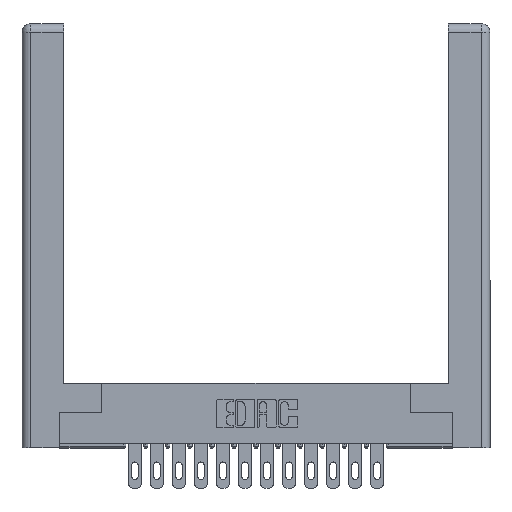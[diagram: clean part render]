
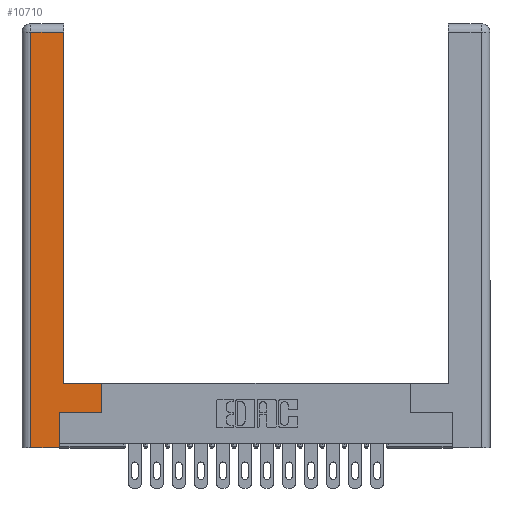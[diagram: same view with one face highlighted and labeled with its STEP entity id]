
A CAD part, top view. The second image highlights one B-rep face of the part: STEP entity #10710.
In plain terms, the highlighted planar face has unit normal (0, 0, 1).
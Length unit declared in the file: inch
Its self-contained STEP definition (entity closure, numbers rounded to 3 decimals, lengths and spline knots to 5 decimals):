
#249 = LINE ( 'NONE', #18550, #14050 ) ;
#365 = LINE ( 'NONE', #11459, #13001 ) ;
#536 = ORIENTED_EDGE ( 'NONE', *, *, #5729, .T. ) ;
#1111 = LINE ( 'NONE', #8922, #12558 ) ;
#1898 = VECTOR ( 'NONE', #13755, 39.37008 ) ;
#2188 = VERTEX_POINT ( 'NONE', #16757 ) ;
#2246 = DIRECTION ( 'NONE',  ( 0., -1., 0. ) ) ;
#2327 = CARTESIAN_POINT ( 'NONE',  ( 0.265, 0.245, 0. ) ) ;
#2480 = EDGE_CURVE ( 'NONE', #4281, #11758, #11964, .T. ) ;
#2519 = CARTESIAN_POINT ( 'NONE',  ( 0.565, 0.45, 0. ) ) ;
#2804 = EDGE_CURVE ( 'NONE', #11758, #7143, #9350, .T. ) ;
#2908 = CARTESIAN_POINT ( 'NONE',  ( 0.565, 0.45, 0. ) ) ;
#3025 = DIRECTION ( 'NONE',  ( -1., 0., 0. ) ) ;
#3849 = LINE ( 'NONE', #11036, #17825 ) ;
#3881 = CARTESIAN_POINT ( 'NONE',  ( 0.295, 2.94, 0. ) ) ;
#3915 = LINE ( 'NONE', #4921, #11590 ) ;
#3989 = LINE ( 'NONE', #2908, #16822 ) ;
#4281 = VERTEX_POINT ( 'NONE', #2519 ) ;
#4641 = ORIENTED_EDGE ( 'NONE', *, *, #2480, .T. ) ;
#4921 = CARTESIAN_POINT ( 'NONE',  ( 0.265, 0., 0. ) ) ;
#5111 = PLANE ( 'NONE',  #7234 ) ;
#5588 = EDGE_CURVE ( 'NONE', #13785, #11558, #3915, .T. ) ;
#5589 = DIRECTION ( 'NONE',  ( 0., 1., 0. ) ) ;
#5644 = VECTOR ( 'NONE', #11297, 39.37008 ) ;
#5729 = EDGE_CURVE ( 'NONE', #11320, #19156, #365, .T. ) ;
#5910 = ORIENTED_EDGE ( 'NONE', *, *, #11909, .T. ) ;
#6810 = DIRECTION ( 'NONE',  ( -1., 0., 0. ) ) ;
#7143 = VERTEX_POINT ( 'NONE', #3881 ) ;
#7176 = ORIENTED_EDGE ( 'NONE', *, *, #2804, .T. ) ;
#7234 = AXIS2_PLACEMENT_3D ( 'NONE', #18779, #11143, #6810 ) ;
#7553 = EDGE_CURVE ( 'NONE', #7143, #2188, #1111, .T. ) ;
#7681 = EDGE_LOOP ( 'NONE', ( #7176, #13729, #11683, #19133, #5910, #536, #16242, #4641 ) ) ;
#7735 = CARTESIAN_POINT ( 'NONE',  ( 0.295, 3., 0. ) ) ;
#8383 = FACE_OUTER_BOUND ( 'NONE', #7681, .T. ) ;
#8732 = CARTESIAN_POINT ( 'NONE',  ( 0.265, 0., 0. ) ) ;
#8922 = CARTESIAN_POINT ( 'NONE',  ( 0.0615, 2.94, 0. ) ) ;
#9350 = LINE ( 'NONE', #7735, #1898 ) ;
#9451 = EDGE_CURVE ( 'NONE', #2188, #13785, #3849, .T. ) ;
#9976 = CARTESIAN_POINT ( 'NONE',  ( 0.295, 0.45, 0. ) ) ;
#9998 = CARTESIAN_POINT ( 'NONE',  ( 0.565, 0.245, 0. ) ) ;
#10078 = DIRECTION ( 'NONE',  ( 1., 0., 0. ) ) ;
#10436 = CARTESIAN_POINT ( 'NONE',  ( 0.0615, 0., 0. ) ) ;
#10710 = ADVANCED_FACE ( 'NONE', ( #8383 ), #5111, .F. ) ;
#11036 = CARTESIAN_POINT ( 'NONE',  ( 0.0615, 0., 0. ) ) ;
#11143 = DIRECTION ( 'NONE',  ( 0., 0., -1. ) ) ;
#11297 = DIRECTION ( 'NONE',  ( -1., 0., 0. ) ) ;
#11320 = VERTEX_POINT ( 'NONE', #2327 ) ;
#11459 = CARTESIAN_POINT ( 'NONE',  ( 0.565, 0.245, 0. ) ) ;
#11558 = VERTEX_POINT ( 'NONE', #8732 ) ;
#11590 = VECTOR ( 'NONE', #16991, 39.37008 ) ;
#11683 = ORIENTED_EDGE ( 'NONE', *, *, #9451, .T. ) ;
#11758 = VERTEX_POINT ( 'NONE', #16873 ) ;
#11909 = EDGE_CURVE ( 'NONE', #11558, #11320, #249, .T. ) ;
#11964 = LINE ( 'NONE', #9976, #5644 ) ;
#12434 = EDGE_CURVE ( 'NONE', #19156, #4281, #3989, .T. ) ;
#12558 = VECTOR ( 'NONE', #3025, 39.37008 ) ;
#13001 = VECTOR ( 'NONE', #10078, 39.37008 ) ;
#13729 = ORIENTED_EDGE ( 'NONE', *, *, #7553, .T. ) ;
#13755 = DIRECTION ( 'NONE',  ( 0., 1., 0. ) ) ;
#13785 = VERTEX_POINT ( 'NONE', #10436 ) ;
#14050 = VECTOR ( 'NONE', #15610, 39.37008 ) ;
#15610 = DIRECTION ( 'NONE',  ( 0., 1., 0. ) ) ;
#16242 = ORIENTED_EDGE ( 'NONE', *, *, #12434, .T. ) ;
#16757 = CARTESIAN_POINT ( 'NONE',  ( 0.0615, 2.94, 0. ) ) ;
#16822 = VECTOR ( 'NONE', #5589, 39.37008 ) ;
#16873 = CARTESIAN_POINT ( 'NONE',  ( 0.295, 0.45, 0. ) ) ;
#16991 = DIRECTION ( 'NONE',  ( 1., 0., 0. ) ) ;
#17825 = VECTOR ( 'NONE', #2246, 39.37008 ) ;
#18550 = CARTESIAN_POINT ( 'NONE',  ( 0.265, 0.245, 0. ) ) ;
#18779 = CARTESIAN_POINT ( 'NONE',  ( 0., 0., 0. ) ) ;
#19133 = ORIENTED_EDGE ( 'NONE', *, *, #5588, .T. ) ;
#19156 = VERTEX_POINT ( 'NONE', #9998 ) ;
